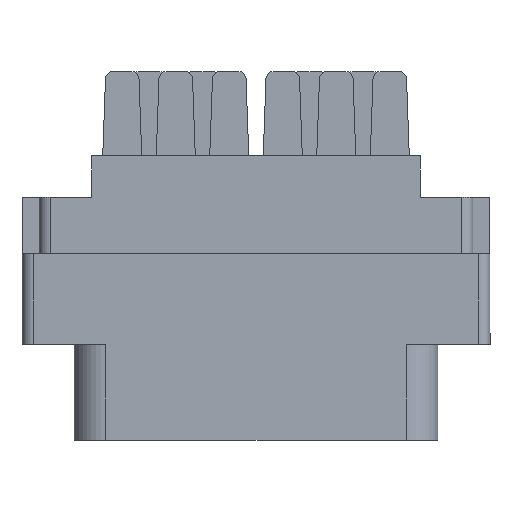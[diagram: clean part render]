
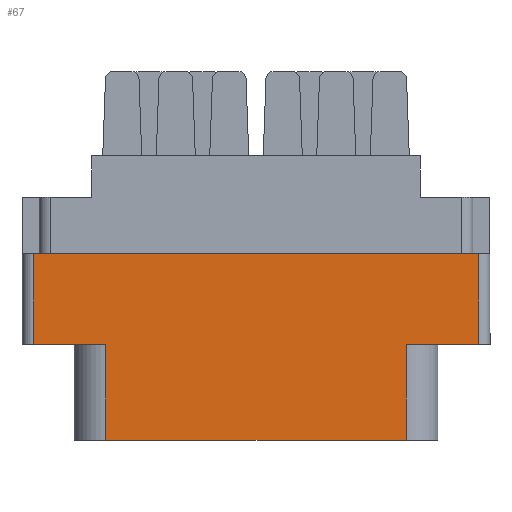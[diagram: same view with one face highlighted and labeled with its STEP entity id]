
A CAD part, front view. The second image highlights one B-rep face of the part: STEP entity #67.
In plain terms, the highlighted planar face has unit normal (0, -1, 0).
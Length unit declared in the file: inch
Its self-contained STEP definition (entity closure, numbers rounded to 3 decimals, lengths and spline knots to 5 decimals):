
#67 = ADVANCED_FACE ( 'NONE', ( #23922 ), #9040, .T. ) ;
#351 = VECTOR ( 'NONE', #6332, 39.37008 ) ;
#411 = DIRECTION ( 'NONE',  ( -1., 0., 0. ) ) ;
#965 = LINE ( 'NONE', #18143, #26919 ) ;
#1559 = LINE ( 'NONE', #19692, #11707 ) ;
#1882 = ORIENTED_EDGE ( 'NONE', *, *, #18067, .F. ) ;
#2496 = VECTOR ( 'NONE', #4893, 39.37008 ) ;
#3125 = DIRECTION ( 'NONE',  ( 1., 0., 0. ) ) ;
#3511 = CARTESIAN_POINT ( 'NONE',  ( -0.42052, -0.343, -0.798 ) ) ;
#3816 = CARTESIAN_POINT ( 'NONE',  ( -0.656, -0.343, -0.798 ) ) ;
#4187 = EDGE_CURVE ( 'NONE', #6175, #11537, #965, .T. ) ;
#4296 = DIRECTION ( 'NONE',  ( 0., -1., 0. ) ) ;
#4752 = CARTESIAN_POINT ( 'NONE',  ( 0.42052, -0.343, -0.529 ) ) ;
#4893 = DIRECTION ( 'NONE',  ( 0., 0., 1. ) ) ;
#5781 = VECTOR ( 'NONE', #10694, 39.37008 ) ;
#5926 = VERTEX_POINT ( 'NONE', #12569 ) ;
#6175 = VERTEX_POINT ( 'NONE', #10571 ) ;
#6332 = DIRECTION ( 'NONE',  ( 0., 0., 1. ) ) ;
#6601 = ORIENTED_EDGE ( 'NONE', *, *, #21491, .T. ) ;
#6863 = CARTESIAN_POINT ( 'NONE',  ( 0., -0.343, -0.529 ) ) ;
#6898 = EDGE_CURVE ( 'NONE', #14274, #25945, #13733, .T. ) ;
#8881 = DIRECTION ( 'NONE',  ( 0., 0., -1. ) ) ;
#8884 = CARTESIAN_POINT ( 'NONE',  ( -0.656, -0.343, -0.798 ) ) ;
#9013 = VECTOR ( 'NONE', #22828, 39.37008 ) ;
#9040 = PLANE ( 'NONE',  #20732 ) ;
#9410 = VERTEX_POINT ( 'NONE', #24547 ) ;
#9521 = VERTEX_POINT ( 'NONE', #18484 ) ;
#10158 = EDGE_LOOP ( 'NONE', ( #1882, #6601, #17479, #15111, #20411, #15656, #25375, #10666 ) ) ;
#10571 = CARTESIAN_POINT ( 'NONE',  ( -0.624, -0.343, -0.529 ) ) ;
#10666 = ORIENTED_EDGE ( 'NONE', *, *, #15679, .T. ) ;
#10694 = DIRECTION ( 'NONE',  ( 1., 0., 0. ) ) ;
#10904 = CARTESIAN_POINT ( 'NONE',  ( 0.624, -0.343, -0.529 ) ) ;
#11537 = VERTEX_POINT ( 'NONE', #16745 ) ;
#11707 = VECTOR ( 'NONE', #12443, 39.37008 ) ;
#12443 = DIRECTION ( 'NONE',  ( 0., 0., -1. ) ) ;
#12569 = CARTESIAN_POINT ( 'NONE',  ( 0.624, -0.343, -0.274 ) ) ;
#13018 = EDGE_CURVE ( 'NONE', #11537, #9410, #28213, .T. ) ;
#13066 = VECTOR ( 'NONE', #8881, 39.37008 ) ;
#13733 = LINE ( 'NONE', #6863, #14362 ) ;
#14274 = VERTEX_POINT ( 'NONE', #10904 ) ;
#14362 = VECTOR ( 'NONE', #411, 39.37008 ) ;
#14845 = LINE ( 'NONE', #3816, #5781 ) ;
#15111 = ORIENTED_EDGE ( 'NONE', *, *, #13018, .T. ) ;
#15656 = ORIENTED_EDGE ( 'NONE', *, *, #15826, .T. ) ;
#15679 = EDGE_CURVE ( 'NONE', #14274, #5926, #18900, .T. ) ;
#15826 = EDGE_CURVE ( 'NONE', #26914, #25945, #24235, .T. ) ;
#16745 = CARTESIAN_POINT ( 'NONE',  ( -0.42052, -0.343, -0.529 ) ) ;
#17422 = CARTESIAN_POINT ( 'NONE',  ( 0., -0.343, -0.274 ) ) ;
#17479 = ORIENTED_EDGE ( 'NONE', *, *, #4187, .T. ) ;
#17618 = CARTESIAN_POINT ( 'NONE',  ( 0.42052, -0.343, -0.529 ) ) ;
#18067 = EDGE_CURVE ( 'NONE', #9521, #5926, #22414, .T. ) ;
#18143 = CARTESIAN_POINT ( 'NONE',  ( 0., -0.343, -0.529 ) ) ;
#18484 = CARTESIAN_POINT ( 'NONE',  ( -0.624, -0.343, -0.274 ) ) ;
#18900 = LINE ( 'NONE', #23660, #351 ) ;
#19692 = CARTESIAN_POINT ( 'NONE',  ( -0.624, -0.343, -0.798 ) ) ;
#20411 = ORIENTED_EDGE ( 'NONE', *, *, #22654, .T. ) ;
#20563 = CARTESIAN_POINT ( 'NONE',  ( 0.42052, -0.343, -0.798 ) ) ;
#20732 = AXIS2_PLACEMENT_3D ( 'NONE', #8884, #4296, #26362 ) ;
#21491 = EDGE_CURVE ( 'NONE', #9521, #6175, #1559, .T. ) ;
#22414 = LINE ( 'NONE', #17422, #9013 ) ;
#22654 = EDGE_CURVE ( 'NONE', #9410, #26914, #14845, .T. ) ;
#22828 = DIRECTION ( 'NONE',  ( 1., 0., 0. ) ) ;
#23660 = CARTESIAN_POINT ( 'NONE',  ( 0.624, -0.343, -0.798 ) ) ;
#23922 = FACE_OUTER_BOUND ( 'NONE', #10158, .T. ) ;
#24235 = LINE ( 'NONE', #17618, #2496 ) ;
#24547 = CARTESIAN_POINT ( 'NONE',  ( -0.42052, -0.343, -0.798 ) ) ;
#25375 = ORIENTED_EDGE ( 'NONE', *, *, #6898, .F. ) ;
#25945 = VERTEX_POINT ( 'NONE', #4752 ) ;
#26362 = DIRECTION ( 'NONE',  ( 0., 0., -1. ) ) ;
#26914 = VERTEX_POINT ( 'NONE', #20563 ) ;
#26919 = VECTOR ( 'NONE', #3125, 39.37008 ) ;
#28213 = LINE ( 'NONE', #3511, #13066 ) ;
